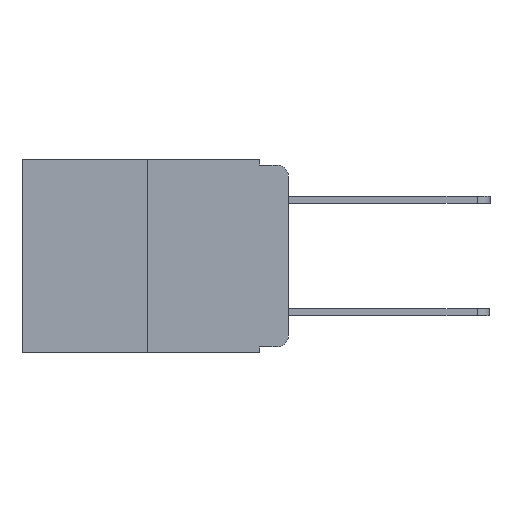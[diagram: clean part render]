
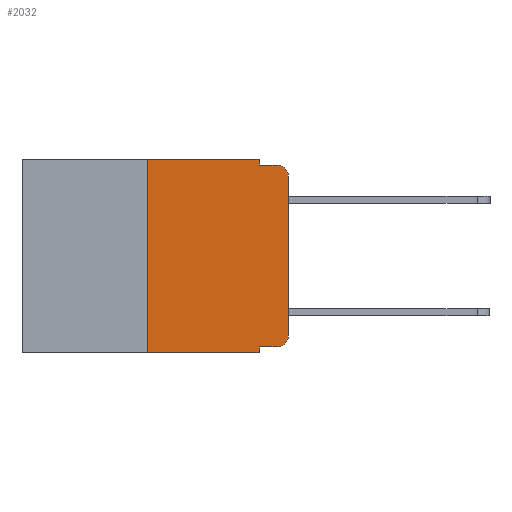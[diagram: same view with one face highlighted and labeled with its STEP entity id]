
A CAD part, left-side view. The second image highlights one B-rep face of the part: STEP entity #2032.
In plain terms, the highlighted planar face has unit normal (-1, 0, 0).
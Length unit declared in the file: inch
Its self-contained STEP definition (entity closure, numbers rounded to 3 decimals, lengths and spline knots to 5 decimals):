
#183 = EDGE_CURVE ( 'NONE', #14784, #5963, #4120, .T. ) ;
#434 = CARTESIAN_POINT ( 'NONE',  ( 0., 0.051, 0. ) ) ;
#642 = VECTOR ( 'NONE', #5036, 39.37008 ) ;
#1070 = EDGE_CURVE ( 'NONE', #9767, #4680, #4519, .T. ) ;
#1180 = DIRECTION ( 'NONE',  ( 1., 0., 0. ) ) ;
#1230 = VERTEX_POINT ( 'NONE', #5184 ) ;
#1346 = ORIENTED_EDGE ( 'NONE', *, *, #1070, .F. ) ;
#1505 = CARTESIAN_POINT ( 'NONE',  ( 0., 0., 0. ) ) ;
#2032 = ADVANCED_FACE ( 'NONE', ( #12213 ), #5537, .F. ) ;
#2104 = CARTESIAN_POINT ( 'NONE',  ( 0., 0.473, 0. ) ) ;
#2292 = CARTESIAN_POINT ( 'NONE',  ( 0., 0.473, 0. ) ) ;
#2560 = LINE ( 'NONE', #6890, #16249 ) ;
#2885 = DIRECTION ( 'NONE',  ( 0., 0., 1. ) ) ;
#3288 = EDGE_CURVE ( 'NONE', #8026, #7818, #17252, .T. ) ;
#3472 = DIRECTION ( 'NONE',  ( 0., -1., 0. ) ) ;
#3692 = VECTOR ( 'NONE', #17475, 39.37008 ) ;
#3803 = VECTOR ( 'NONE', #2885, 39.37008 ) ;
#4120 = CIRCLE ( 'NONE', #8918, 0.02 ) ;
#4125 = EDGE_CURVE ( 'NONE', #4680, #8026, #5287, .T. ) ;
#4277 = CARTESIAN_POINT ( 'NONE',  ( 0., 0.25, 0. ) ) ;
#4346 = LINE ( 'NONE', #14596, #642 ) ;
#4519 = LINE ( 'NONE', #16316, #7770 ) ;
#4680 = VERTEX_POINT ( 'NONE', #4277 ) ;
#4729 = VERTEX_POINT ( 'NONE', #13766 ) ;
#4851 = DIRECTION ( 'NONE',  ( -1., 0., 0. ) ) ;
#4988 = LINE ( 'NONE', #7430, #15449 ) ;
#5036 = DIRECTION ( 'NONE',  ( 0., -1., 0. ) ) ;
#5184 = CARTESIAN_POINT ( 'NONE',  ( 0., 0.051, -0.333 ) ) ;
#5287 = LINE ( 'NONE', #2104, #16582 ) ;
#5537 = PLANE ( 'NONE',  #16864 ) ;
#5706 = VERTEX_POINT ( 'NONE', #11525 ) ;
#5730 = CARTESIAN_POINT ( 'NONE',  ( 0., 0.02, -0.313 ) ) ;
#5791 = DIRECTION ( 'NONE',  ( 0., 0., -1. ) ) ;
#5963 = VERTEX_POINT ( 'NONE', #17045 ) ;
#6192 = EDGE_CURVE ( 'NONE', #1230, #14306, #7372, .T. ) ;
#6585 = DIRECTION ( 'NONE',  ( 0., 0., -1. ) ) ;
#6890 = CARTESIAN_POINT ( 'NONE',  ( 0., 0.473, -0.343 ) ) ;
#6970 = EDGE_CURVE ( 'NONE', #9767, #14306, #2560, .T. ) ;
#7372 = LINE ( 'NONE', #434, #3692 ) ;
#7430 = CARTESIAN_POINT ( 'NONE',  ( 0., 0.051, -0.333 ) ) ;
#7770 = VECTOR ( 'NONE', #16727, 39.37008 ) ;
#7818 = VERTEX_POINT ( 'NONE', #16259 ) ;
#8026 = VERTEX_POINT ( 'NONE', #11574 ) ;
#8202 = CARTESIAN_POINT ( 'NONE',  ( 0., 0.02, -0.333 ) ) ;
#8502 = ORIENTED_EDGE ( 'NONE', *, *, #3288, .F. ) ;
#8682 = ORIENTED_EDGE ( 'NONE', *, *, #183, .T. ) ;
#8918 = AXIS2_PLACEMENT_3D ( 'NONE', #5730, #16358, #5791 ) ;
#8937 = EDGE_LOOP ( 'NONE', ( #16942, #11918, #17171, #8502, #16963, #1346, #10412, #12148, #13832, #8682 ) ) ;
#9068 = AXIS2_PLACEMENT_3D ( 'NONE', #13062, #4851, #14415 ) ;
#9729 = EDGE_CURVE ( 'NONE', #7818, #5706, #4346, .T. ) ;
#9767 = VERTEX_POINT ( 'NONE', #13352 ) ;
#9941 = CARTESIAN_POINT ( 'NONE',  ( 0., 0.051, -0.343 ) ) ;
#10412 = ORIENTED_EDGE ( 'NONE', *, *, #6970, .T. ) ;
#10474 = VECTOR ( 'NONE', #17071, 39.37008 ) ;
#11525 = CARTESIAN_POINT ( 'NONE',  ( 0., 0.02, -0.01 ) ) ;
#11574 = CARTESIAN_POINT ( 'NONE',  ( 0., 0.051, 0. ) ) ;
#11890 = EDGE_CURVE ( 'NONE', #4729, #5706, #12013, .T. ) ;
#11918 = ORIENTED_EDGE ( 'NONE', *, *, #11890, .T. ) ;
#12013 = CIRCLE ( 'NONE', #9068, 0.02 ) ;
#12077 = DIRECTION ( 'NONE',  ( 0., -1., 0. ) ) ;
#12123 = EDGE_CURVE ( 'NONE', #5963, #4729, #14725, .T. ) ;
#12148 = ORIENTED_EDGE ( 'NONE', *, *, #6192, .F. ) ;
#12213 = FACE_OUTER_BOUND ( 'NONE', #8937, .T. ) ;
#13062 = CARTESIAN_POINT ( 'NONE',  ( 0., 0.02, -0.03 ) ) ;
#13352 = CARTESIAN_POINT ( 'NONE',  ( 0., 0.25, -0.343 ) ) ;
#13766 = CARTESIAN_POINT ( 'NONE',  ( 0., 0., -0.03 ) ) ;
#13832 = ORIENTED_EDGE ( 'NONE', *, *, #14426, .T. ) ;
#14206 = DIRECTION ( 'NONE',  ( 0., -1., 0. ) ) ;
#14306 = VERTEX_POINT ( 'NONE', #9941 ) ;
#14415 = DIRECTION ( 'NONE',  ( 0., 0., -1. ) ) ;
#14426 = EDGE_CURVE ( 'NONE', #1230, #14784, #4988, .T. ) ;
#14596 = CARTESIAN_POINT ( 'NONE',  ( 0., 0.051, -0.01 ) ) ;
#14725 = LINE ( 'NONE', #1505, #3803 ) ;
#14784 = VERTEX_POINT ( 'NONE', #8202 ) ;
#15449 = VECTOR ( 'NONE', #14206, 39.37008 ) ;
#16249 = VECTOR ( 'NONE', #12077, 39.37008 ) ;
#16259 = CARTESIAN_POINT ( 'NONE',  ( 0., 0.051, -0.01 ) ) ;
#16316 = CARTESIAN_POINT ( 'NONE',  ( 0., 0.25, 0. ) ) ;
#16358 = DIRECTION ( 'NONE',  ( -1., 0., 0. ) ) ;
#16582 = VECTOR ( 'NONE', #3472, 39.37008 ) ;
#16727 = DIRECTION ( 'NONE',  ( 0., 0., 1. ) ) ;
#16864 = AXIS2_PLACEMENT_3D ( 'NONE', #2292, #1180, #6585 ) ;
#16942 = ORIENTED_EDGE ( 'NONE', *, *, #12123, .T. ) ;
#16963 = ORIENTED_EDGE ( 'NONE', *, *, #4125, .F. ) ;
#17045 = CARTESIAN_POINT ( 'NONE',  ( 0., 0., -0.313 ) ) ;
#17071 = DIRECTION ( 'NONE',  ( 0., 0., -1. ) ) ;
#17171 = ORIENTED_EDGE ( 'NONE', *, *, #9729, .F. ) ;
#17252 = LINE ( 'NONE', #17323, #10474 ) ;
#17323 = CARTESIAN_POINT ( 'NONE',  ( 0., 0.051, 0. ) ) ;
#17475 = DIRECTION ( 'NONE',  ( 0., 0., -1. ) ) ;
